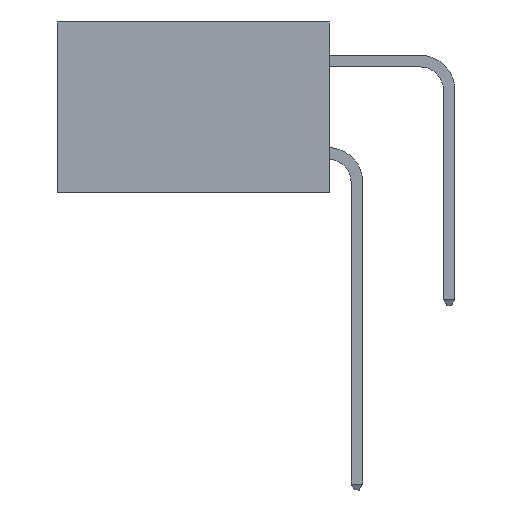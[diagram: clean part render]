
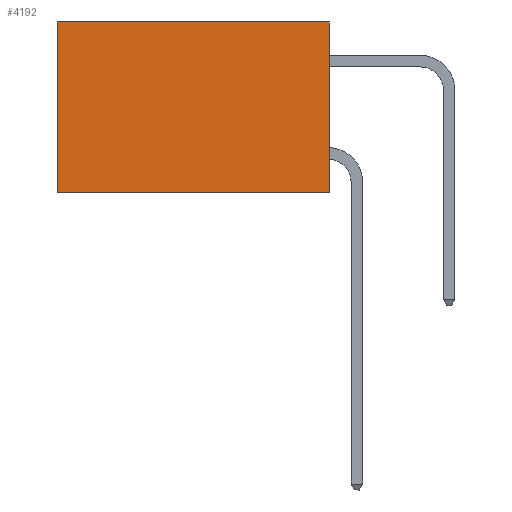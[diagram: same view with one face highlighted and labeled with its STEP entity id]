
A CAD part, left-side view. The second image highlights one B-rep face of the part: STEP entity #4192.
In plain terms, the highlighted planar face has unit normal (-1, 0, 0).
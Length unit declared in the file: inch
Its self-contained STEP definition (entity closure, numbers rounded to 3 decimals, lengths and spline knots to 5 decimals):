
#967 = ORIENTED_EDGE ( 'NONE', *, *, #6886, .F. ) ;
#1407 = CARTESIAN_POINT ( 'NONE',  ( 0.277, 0., -0.37 ) ) ;
#2123 = ORIENTED_EDGE ( 'NONE', *, *, #5434, .F. ) ;
#2149 = EDGE_CURVE ( 'NONE', #5668, #11440, #10088, .T. ) ;
#2216 = VERTEX_POINT ( 'NONE', #5568 ) ;
#2351 = AXIS2_PLACEMENT_3D ( 'NONE', #1407, #7927, #8641 ) ;
#2428 = LINE ( 'NONE', #9223, #8552 ) ;
#2499 = LINE ( 'NONE', #9159, #9933 ) ;
#3033 = EDGE_CURVE ( 'NONE', #10365, #5668, #2499, .T. ) ;
#3410 = CARTESIAN_POINT ( 'NONE',  ( 0.277, 0.59, -0.37 ) ) ;
#3726 = VECTOR ( 'NONE', #6603, 39.37008 ) ;
#4192 = ADVANCED_FACE ( 'NONE', ( #7643 ), #7873, .F. ) ;
#5434 = EDGE_CURVE ( 'NONE', #2216, #11440, #2428, .T. ) ;
#5568 = CARTESIAN_POINT ( 'NONE',  ( 0.277, 0., -0.37 ) ) ;
#5637 = ORIENTED_EDGE ( 'NONE', *, *, #3033, .T. ) ;
#5668 = VERTEX_POINT ( 'NONE', #5879 ) ;
#5879 = CARTESIAN_POINT ( 'NONE',  ( 0.277, 0.59, 0. ) ) ;
#6603 = DIRECTION ( 'NONE',  ( 0., 0., -1. ) ) ;
#6615 = CARTESIAN_POINT ( 'NONE',  ( 0.277, 0., -0.37 ) ) ;
#6765 = EDGE_LOOP ( 'NONE', ( #6957, #2123, #967, #5637 ) ) ;
#6792 = DIRECTION ( 'NONE',  ( 0., 1., 0. ) ) ;
#6886 = EDGE_CURVE ( 'NONE', #10365, #2216, #7860, .T. ) ;
#6957 = ORIENTED_EDGE ( 'NONE', *, *, #2149, .T. ) ;
#7643 = FACE_OUTER_BOUND ( 'NONE', #6765, .T. ) ;
#7846 = VECTOR ( 'NONE', #10486, 39.37008 ) ;
#7860 = LINE ( 'NONE', #6615, #3726 ) ;
#7873 = PLANE ( 'NONE',  #2351 ) ;
#7927 = DIRECTION ( 'NONE',  ( 1., 0., 0. ) ) ;
#8552 = VECTOR ( 'NONE', #9256, 39.37008 ) ;
#8641 = DIRECTION ( 'NONE',  ( 0., 0., -1. ) ) ;
#9159 = CARTESIAN_POINT ( 'NONE',  ( 0.277, 0., 0. ) ) ;
#9223 = CARTESIAN_POINT ( 'NONE',  ( 0.277, 0., -0.37 ) ) ;
#9256 = DIRECTION ( 'NONE',  ( 0., 1., 0. ) ) ;
#9933 = VECTOR ( 'NONE', #6792, 39.37008 ) ;
#10088 = LINE ( 'NONE', #10098, #7846 ) ;
#10098 = CARTESIAN_POINT ( 'NONE',  ( 0.277, 0.59, -0.37 ) ) ;
#10365 = VERTEX_POINT ( 'NONE', #10779 ) ;
#10486 = DIRECTION ( 'NONE',  ( 0., 0., -1. ) ) ;
#10779 = CARTESIAN_POINT ( 'NONE',  ( 0.277, 0., 0. ) ) ;
#11440 = VERTEX_POINT ( 'NONE', #3410 ) ;
